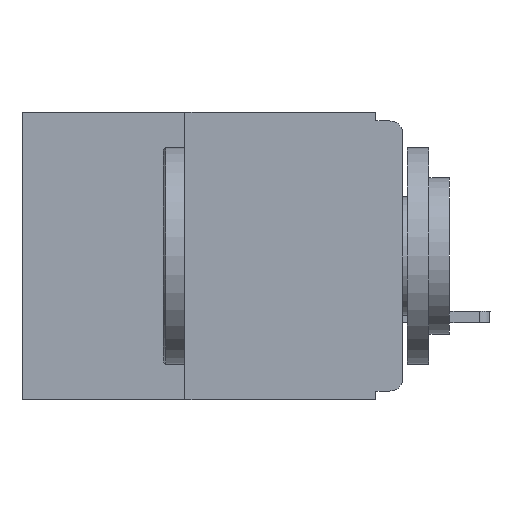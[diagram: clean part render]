
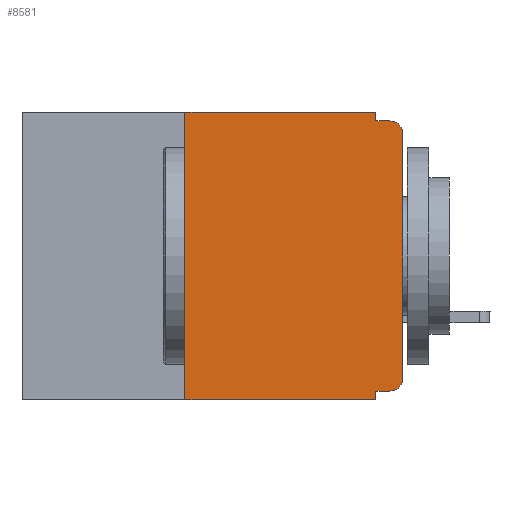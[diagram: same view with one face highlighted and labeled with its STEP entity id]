
A CAD part, left-side view. The second image highlights one B-rep face of the part: STEP entity #8581.
In plain terms, the highlighted planar face has unit normal (-1, 0, 0).
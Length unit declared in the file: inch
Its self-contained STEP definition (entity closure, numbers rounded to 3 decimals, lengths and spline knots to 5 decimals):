
#218 = CARTESIAN_POINT ( 'NONE',  ( 0., 0.031, -0.01 ) ) ;
#303 = CARTESIAN_POINT ( 'NONE',  ( 0., 0.015, -0.32 ) ) ;
#388 = ORIENTED_EDGE ( 'NONE', *, *, #3179, .T. ) ;
#523 = ORIENTED_EDGE ( 'NONE', *, *, #16230, .T. ) ;
#683 = DIRECTION ( 'NONE',  ( 0., 0., -1. ) ) ;
#685 = CARTESIAN_POINT ( 'NONE',  ( 0., 0., -0.025 ) ) ;
#882 = LINE ( 'NONE', #1425, #7444 ) ;
#1095 = DIRECTION ( 'NONE',  ( 0., 0., 1. ) ) ;
#1237 = CIRCLE ( 'NONE', #13805, 0.015 ) ;
#1425 = CARTESIAN_POINT ( 'NONE',  ( 0., 0., -0.01 ) ) ;
#2172 = DIRECTION ( 'NONE',  ( 0., -1., 0. ) ) ;
#2228 = CARTESIAN_POINT ( 'NONE',  ( 0., 0.437, 0. ) ) ;
#2452 = DIRECTION ( 'NONE',  ( -1., 0., 0. ) ) ;
#2655 = EDGE_CURVE ( 'NONE', #16886, #3143, #882, .T. ) ;
#2704 = VECTOR ( 'NONE', #8505, 39.37008 ) ;
#3087 = CARTESIAN_POINT ( 'NONE',  ( 0., 0.25, 0. ) ) ;
#3143 = VERTEX_POINT ( 'NONE', #3373 ) ;
#3179 = EDGE_CURVE ( 'NONE', #10211, #3143, #10770, .T. ) ;
#3241 = DIRECTION ( 'NONE',  ( 0., 0., 1. ) ) ;
#3373 = CARTESIAN_POINT ( 'NONE',  ( 0., 0.015, -0.01 ) ) ;
#3395 = LINE ( 'NONE', #2228, #12242 ) ;
#3884 = VECTOR ( 'NONE', #11647, 39.37008 ) ;
#4013 = CARTESIAN_POINT ( 'NONE',  ( 0., 0., -0.32 ) ) ;
#4132 = AXIS2_PLACEMENT_3D ( 'NONE', #8938, #2452, #16977 ) ;
#4631 = PLANE ( 'NONE',  #12926 ) ;
#4676 = VERTEX_POINT ( 'NONE', #3087 ) ;
#4711 = LINE ( 'NONE', #9827, #9690 ) ;
#4777 = VECTOR ( 'NONE', #11127, 39.37008 ) ;
#4799 = ORIENTED_EDGE ( 'NONE', *, *, #15314, .T. ) ;
#5090 = VECTOR ( 'NONE', #17073, 39.37008 ) ;
#5388 = DIRECTION ( 'NONE',  ( 0., -1., 0. ) ) ;
#6178 = LINE ( 'NONE', #16445, #2704 ) ;
#6314 = CARTESIAN_POINT ( 'NONE',  ( 0., 0.25, -0.33 ) ) ;
#6962 = ORIENTED_EDGE ( 'NONE', *, *, #14582, .F. ) ;
#7087 = CARTESIAN_POINT ( 'NONE',  ( 0., 0.015, -0.305 ) ) ;
#7432 = ORIENTED_EDGE ( 'NONE', *, *, #16796, .F. ) ;
#7435 = ORIENTED_EDGE ( 'NONE', *, *, #2655, .F. ) ;
#7444 = VECTOR ( 'NONE', #5388, 39.37008 ) ;
#7478 = DIRECTION ( 'NONE',  ( 1., 0., 0. ) ) ;
#7758 = CARTESIAN_POINT ( 'NONE',  ( 0., 0.031, 0. ) ) ;
#7836 = ORIENTED_EDGE ( 'NONE', *, *, #11131, .F. ) ;
#8057 = LINE ( 'NONE', #9867, #4777 ) ;
#8065 = VERTEX_POINT ( 'NONE', #12159 ) ;
#8505 = DIRECTION ( 'NONE',  ( 0., 0., -1. ) ) ;
#8581 = ADVANCED_FACE ( 'NONE', ( #10795 ), #4631, .F. ) ;
#8744 = ORIENTED_EDGE ( 'NONE', *, *, #10915, .T. ) ;
#8938 = CARTESIAN_POINT ( 'NONE',  ( 0., 0.015, -0.025 ) ) ;
#9255 = VERTEX_POINT ( 'NONE', #9263 ) ;
#9263 = CARTESIAN_POINT ( 'NONE',  ( 0., 0., -0.305 ) ) ;
#9676 = DIRECTION ( 'NONE',  ( -1., 0., 0. ) ) ;
#9690 = VECTOR ( 'NONE', #3241, 39.37008 ) ;
#9827 = CARTESIAN_POINT ( 'NONE',  ( 0., 0., 0. ) ) ;
#9867 = CARTESIAN_POINT ( 'NONE',  ( 0., 0.031, -0.33 ) ) ;
#10187 = EDGE_CURVE ( 'NONE', #12436, #16886, #6178, .T. ) ;
#10211 = VERTEX_POINT ( 'NONE', #685 ) ;
#10694 = VECTOR ( 'NONE', #1095, 39.37008 ) ;
#10770 = CIRCLE ( 'NONE', #4132, 0.015 ) ;
#10795 = FACE_OUTER_BOUND ( 'NONE', #11339, .T. ) ;
#10865 = CARTESIAN_POINT ( 'NONE',  ( 0., 0.25, -0.33 ) ) ;
#10915 = EDGE_CURVE ( 'NONE', #9255, #10211, #4711, .T. ) ;
#11127 = DIRECTION ( 'NONE',  ( 0., 0., -1. ) ) ;
#11131 = EDGE_CURVE ( 'NONE', #13786, #4676, #13353, .T. ) ;
#11339 = EDGE_LOOP ( 'NONE', ( #8744, #388, #7435, #14937, #12278, #7836, #523, #6962, #7432, #4799 ) ) ;
#11647 = DIRECTION ( 'NONE',  ( 0., -1., 0. ) ) ;
#12159 = CARTESIAN_POINT ( 'NONE',  ( 0., 0.031, -0.33 ) ) ;
#12242 = VECTOR ( 'NONE', #2172, 39.37008 ) ;
#12278 = ORIENTED_EDGE ( 'NONE', *, *, #13304, .F. ) ;
#12436 = VERTEX_POINT ( 'NONE', #7758 ) ;
#12589 = CARTESIAN_POINT ( 'NONE',  ( 0., 0.437, 0. ) ) ;
#12922 = CARTESIAN_POINT ( 'NONE',  ( 0., 0.437, -0.33 ) ) ;
#12926 = AXIS2_PLACEMENT_3D ( 'NONE', #12589, #7478, #14191 ) ;
#13304 = EDGE_CURVE ( 'NONE', #4676, #12436, #3395, .T. ) ;
#13353 = LINE ( 'NONE', #6314, #10694 ) ;
#13786 = VERTEX_POINT ( 'NONE', #10865 ) ;
#13801 = VERTEX_POINT ( 'NONE', #303 ) ;
#13805 = AXIS2_PLACEMENT_3D ( 'NONE', #7087, #9676, #683 ) ;
#14191 = DIRECTION ( 'NONE',  ( 0., 0., -1. ) ) ;
#14357 = CARTESIAN_POINT ( 'NONE',  ( 0., 0.031, -0.32 ) ) ;
#14582 = EDGE_CURVE ( 'NONE', #16221, #8065, #8057, .T. ) ;
#14937 = ORIENTED_EDGE ( 'NONE', *, *, #10187, .F. ) ;
#15314 = EDGE_CURVE ( 'NONE', #13801, #9255, #1237, .T. ) ;
#15419 = LINE ( 'NONE', #4013, #5090 ) ;
#16221 = VERTEX_POINT ( 'NONE', #14357 ) ;
#16230 = EDGE_CURVE ( 'NONE', #13786, #8065, #16287, .T. ) ;
#16287 = LINE ( 'NONE', #12922, #3884 ) ;
#16445 = CARTESIAN_POINT ( 'NONE',  ( 0., 0.031, 0. ) ) ;
#16796 = EDGE_CURVE ( 'NONE', #13801, #16221, #15419, .T. ) ;
#16886 = VERTEX_POINT ( 'NONE', #218 ) ;
#16977 = DIRECTION ( 'NONE',  ( 0., 0., -1. ) ) ;
#17073 = DIRECTION ( 'NONE',  ( 0., 1., 0. ) ) ;
